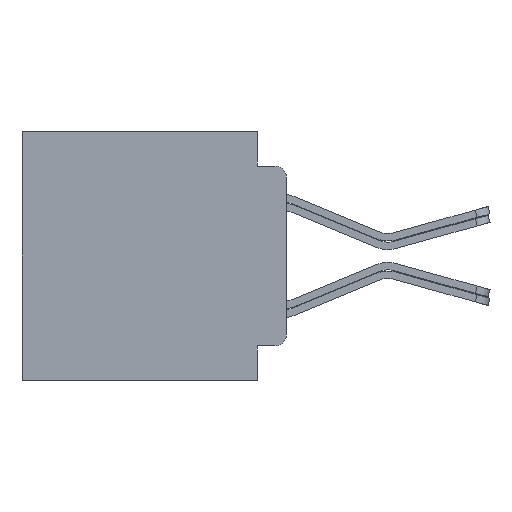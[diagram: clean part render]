
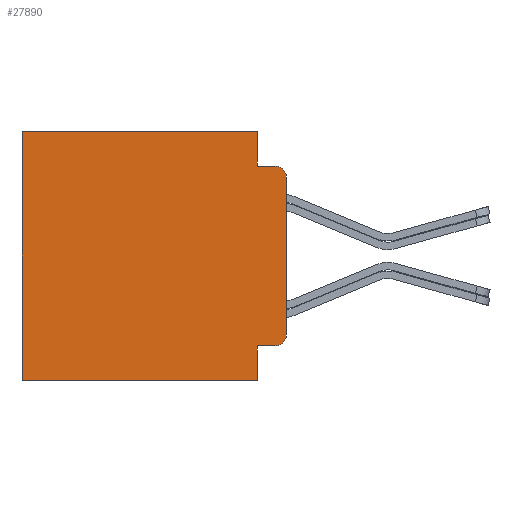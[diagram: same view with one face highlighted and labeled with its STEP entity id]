
A CAD part, left-side view. The second image highlights one B-rep face of the part: STEP entity #27890.
In plain terms, the highlighted planar face has unit normal (-1, 0, 0).
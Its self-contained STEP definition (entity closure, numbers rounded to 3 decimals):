
#47 = CARTESIAN_POINT ( 'NONE',  ( -67.462, 1.295, 0. ) ) ;
#167 = VECTOR ( 'NONE', #12057, 1000. ) ;
#713 = DIRECTION ( 'NONE',  ( 0., 0., -1. ) ) ;
#960 = ORIENTED_EDGE ( 'NONE', *, *, #28024, .T. ) ;
#1217 = EDGE_CURVE ( 'NONE', #16504, #26526, #20164, .T. ) ;
#1563 = LINE ( 'NONE', #1945, #21119 ) ;
#1945 = CARTESIAN_POINT ( 'NONE',  ( -67.462, 0., -5.486 ) ) ;
#2370 = ORIENTED_EDGE ( 'NONE', *, *, #17193, .T. ) ;
#2556 = PLANE ( 'NONE',  #13656 ) ;
#3108 = VECTOR ( 'NONE', #11210, 1000. ) ;
#4334 = CARTESIAN_POINT ( 'NONE',  ( -67.462, 1.295, -5.486 ) ) ;
#4514 = CARTESIAN_POINT ( 'NONE',  ( -67.462, 1.295, -3.975 ) ) ;
#4667 = DIRECTION ( 'NONE',  ( 0., 0., -1. ) ) ;
#4780 = DIRECTION ( 'NONE',  ( 1., 0., 0. ) ) ;
#4848 = EDGE_CURVE ( 'NONE', #16504, #21410, #16885, .T. ) ;
#4964 = CARTESIAN_POINT ( 'NONE',  ( -67.462, 0., -5.486 ) ) ;
#6458 = CIRCLE ( 'NONE', #9635, 0.508 ) ;
#7084 = LINE ( 'NONE', #16139, #167 ) ;
#7262 = DIRECTION ( 'NONE',  ( 0., 0., -1. ) ) ;
#7542 = DIRECTION ( 'NONE',  ( 0., 0., -1. ) ) ;
#7905 = VERTEX_POINT ( 'NONE', #28070 ) ;
#7944 = ORIENTED_EDGE ( 'NONE', *, *, #14673, .T. ) ;
#8049 = VECTOR ( 'NONE', #13692, 1000. ) ;
#8343 = EDGE_CURVE ( 'NONE', #8969, #20296, #7084, .T. ) ;
#8799 = VECTOR ( 'NONE', #26751, 1000. ) ;
#8969 = VERTEX_POINT ( 'NONE', #12602 ) ;
#9635 = AXIS2_PLACEMENT_3D ( 'NONE', #18255, #20464, #7542 ) ;
#9862 = EDGE_CURVE ( 'NONE', #22746, #8969, #18987, .T. ) ;
#10653 = CARTESIAN_POINT ( 'NONE',  ( -67.462, 11.684, 5.486 ) ) ;
#11210 = DIRECTION ( 'NONE',  ( 0., 0., -1. ) ) ;
#11350 = LINE ( 'NONE', #4964, #3108 ) ;
#12057 = DIRECTION ( 'NONE',  ( 0., -1., 0. ) ) ;
#12102 = ORIENTED_EDGE ( 'NONE', *, *, #27002, .F. ) ;
#12602 = CARTESIAN_POINT ( 'NONE',  ( -67.462, 1.295, 3.975 ) ) ;
#12753 = EDGE_CURVE ( 'NONE', #26526, #18854, #15407, .T. ) ;
#13482 = VECTOR ( 'NONE', #14346, 1000. ) ;
#13656 = AXIS2_PLACEMENT_3D ( 'NONE', #22300, #4780, #7262 ) ;
#13692 = DIRECTION ( 'NONE',  ( 0., 0., -1. ) ) ;
#14033 = AXIS2_PLACEMENT_3D ( 'NONE', #21910, #26412, #4667 ) ;
#14346 = DIRECTION ( 'NONE',  ( 0., 0., -1. ) ) ;
#14673 = EDGE_CURVE ( 'NONE', #22746, #24059, #19754, .T. ) ;
#15349 = DIRECTION ( 'NONE',  ( 0., 1., 0. ) ) ;
#15407 = CIRCLE ( 'NONE', #14033, 0.508 ) ;
#16139 = CARTESIAN_POINT ( 'NONE',  ( -67.462, 1.295, 3.975 ) ) ;
#16425 = CARTESIAN_POINT ( 'NONE',  ( -67.462, 0., -3.467 ) ) ;
#16504 = VERTEX_POINT ( 'NONE', #18363 ) ;
#16707 = CARTESIAN_POINT ( 'NONE',  ( -67.462, 11.684, -5.486 ) ) ;
#16885 = LINE ( 'NONE', #47, #17559 ) ;
#17193 = EDGE_CURVE ( 'NONE', #24059, #7905, #28212, .T. ) ;
#17559 = VECTOR ( 'NONE', #713, 1000. ) ;
#17644 = ORIENTED_EDGE ( 'NONE', *, *, #1217, .T. ) ;
#18064 = CARTESIAN_POINT ( 'NONE',  ( -67.462, 1.295, 0. ) ) ;
#18255 = CARTESIAN_POINT ( 'NONE',  ( -67.462, 0.508, 3.467 ) ) ;
#18363 = CARTESIAN_POINT ( 'NONE',  ( -67.462, 1.295, -3.975 ) ) ;
#18598 = EDGE_CURVE ( 'NONE', #18610, #18854, #11350, .T. ) ;
#18610 = VERTEX_POINT ( 'NONE', #22487 ) ;
#18854 = VERTEX_POINT ( 'NONE', #16425 ) ;
#18987 = LINE ( 'NONE', #18064, #8049 ) ;
#19533 = EDGE_LOOP ( 'NONE', ( #17644, #20835, #23481, #960, #20767, #19636, #7944, #2370, #12102, #27549 ) ) ;
#19636 = ORIENTED_EDGE ( 'NONE', *, *, #9862, .F. ) ;
#19754 = LINE ( 'NONE', #22630, #8799 ) ;
#20164 = LINE ( 'NONE', #4514, #28399 ) ;
#20296 = VERTEX_POINT ( 'NONE', #21356 ) ;
#20464 = DIRECTION ( 'NONE',  ( -1., 0., 0. ) ) ;
#20767 = ORIENTED_EDGE ( 'NONE', *, *, #8343, .F. ) ;
#20835 = ORIENTED_EDGE ( 'NONE', *, *, #12753, .T. ) ;
#21119 = VECTOR ( 'NONE', #15349, 1000. ) ;
#21356 = CARTESIAN_POINT ( 'NONE',  ( -67.462, 0.508, 3.975 ) ) ;
#21410 = VERTEX_POINT ( 'NONE', #4334 ) ;
#21536 = FACE_OUTER_BOUND ( 'NONE', #19533, .T. ) ;
#21708 = CARTESIAN_POINT ( 'NONE',  ( -67.462, 1.295, 5.486 ) ) ;
#21910 = CARTESIAN_POINT ( 'NONE',  ( -67.462, 0.508, -3.467 ) ) ;
#22044 = DIRECTION ( 'NONE',  ( 0., -1., 0. ) ) ;
#22300 = CARTESIAN_POINT ( 'NONE',  ( -67.462, 0., -5.486 ) ) ;
#22487 = CARTESIAN_POINT ( 'NONE',  ( -67.462, 0., 3.467 ) ) ;
#22630 = CARTESIAN_POINT ( 'NONE',  ( -67.462, 0., 5.486 ) ) ;
#22746 = VERTEX_POINT ( 'NONE', #21708 ) ;
#23481 = ORIENTED_EDGE ( 'NONE', *, *, #18598, .F. ) ;
#24059 = VERTEX_POINT ( 'NONE', #10653 ) ;
#26412 = DIRECTION ( 'NONE',  ( -1., 0., 0. ) ) ;
#26526 = VERTEX_POINT ( 'NONE', #26772 ) ;
#26751 = DIRECTION ( 'NONE',  ( 0., 1., 0. ) ) ;
#26772 = CARTESIAN_POINT ( 'NONE',  ( -67.462, 0.508, -3.975 ) ) ;
#27002 = EDGE_CURVE ( 'NONE', #21410, #7905, #1563, .T. ) ;
#27549 = ORIENTED_EDGE ( 'NONE', *, *, #4848, .F. ) ;
#27890 = ADVANCED_FACE ( 'NONE', ( #21536 ), #2556, .F. ) ;
#28024 = EDGE_CURVE ( 'NONE', #18610, #20296, #6458, .T. ) ;
#28070 = CARTESIAN_POINT ( 'NONE',  ( -67.462, 11.684, -5.486 ) ) ;
#28212 = LINE ( 'NONE', #16707, #13482 ) ;
#28399 = VECTOR ( 'NONE', #22044, 1000. ) ;
